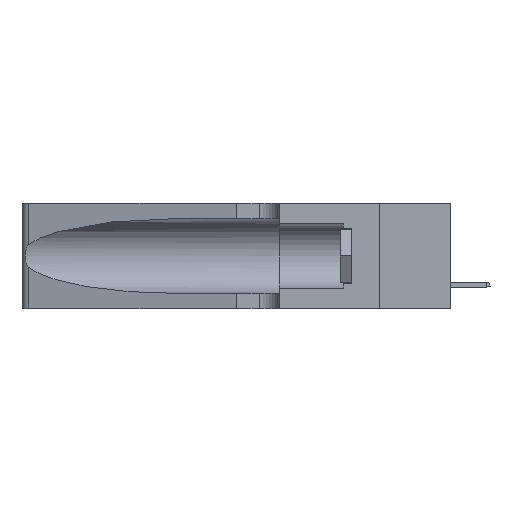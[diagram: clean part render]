
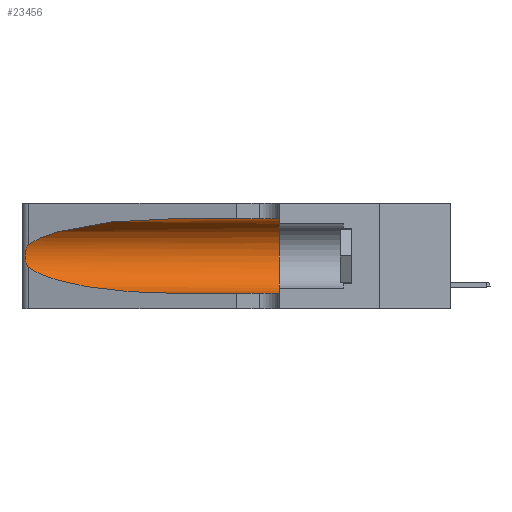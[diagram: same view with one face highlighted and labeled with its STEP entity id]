
A CAD part, left-side view. The second image highlights one B-rep face of the part: STEP entity #23456.
In plain terms, the highlighted cylindrical face has radius 3.308 mm (diameter 6.617 mm), a partial arc.
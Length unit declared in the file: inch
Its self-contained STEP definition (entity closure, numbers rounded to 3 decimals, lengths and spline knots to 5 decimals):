
#141 = CARTESIAN_POINT ( 'NONE',  ( 0.25555, 1.22994, 0.2215 ) ) ;
#647 = CARTESIAN_POINT ( 'NONE',  ( 0.18966, 0.96281, 0.31525 ) ) ;
#2506 = DIRECTION ( 'NONE',  ( 0., -1., 0. ) ) ;
#3282 = AXIS2_PLACEMENT_3D ( 'NONE', #23317, #33966, #10774 ) ;
#3407 = CARTESIAN_POINT ( 'NONE',  ( 0.1305, 1.61858, 0.31525 ) ) ;
#4563 = CARTESIAN_POINT ( 'NONE',  ( 0.1305, 0.72297, 0.31525 ) ) ;
#7041 = CARTESIAN_POINT ( 'NONE',  ( 0.25555, 1.22993, 0.14849 ) ) ;
#7470 = DIRECTION ( 'NONE',  ( 0., 1., 0. ) ) ;
#8236 =( BOUNDED_CURVE ( )  B_SPLINE_CURVE ( 3, ( #4563, #647, #25328, #32719 ),
 .UNSPECIFIED., .F., .T. ) 
 B_SPLINE_CURVE_WITH_KNOTS ( ( 4, 4 ),
 ( 1.5708, 2.84003 ),
 .UNSPECIFIED. ) 
 CURVE ( )  GEOMETRIC_REPRESENTATION_ITEM ( )  RATIONAL_B_SPLINE_CURVE ( ( 1., 0.87, 0.87, 1. ) ) 
 REPRESENTATION_ITEM ( '' )  );
#8951 = ORIENTED_EDGE ( 'NONE', *, *, #14576, .T. ) ;
#10418 = CARTESIAN_POINT ( 'NONE',  ( 0.1305, 1.61858, 0.05475 ) ) ;
#10507 = CARTESIAN_POINT ( 'NONE',  ( 0.25789, 1.23486, 0.15765 ) ) ;
#10774 = DIRECTION ( 'NONE',  ( 0., 0., -1. ) ) ;
#11769 = CARTESIAN_POINT ( 'NONE',  ( 0.1305, 0.35, 0.31525 ) ) ;
#13857 = CARTESIAN_POINT ( 'NONE',  ( 0.25487, 1.22718, 0.14631 ) ) ;
#13956 = CARTESIAN_POINT ( 'NONE',  ( 0.25856, 1.23593, 0.16098 ) ) ;
#14417 = AXIS2_PLACEMENT_3D ( 'NONE', #35677, #7470, #35895 ) ;
#14576 = EDGE_CURVE ( 'NONE', #36772, #32046, #20789, .T. ) ;
#14887 = CARTESIAN_POINT ( 'NONE',  ( 0.25487, 1.22718, 0.22369 ) ) ;
#15373 = CARTESIAN_POINT ( 'NONE',  ( 0.1305, 0.72297, 0.05475 ) ) ;
#15711 = CARTESIAN_POINT ( 'NONE',  ( 0.25487, 1.22718, 0.14631 ) ) ;
#16913 = CARTESIAN_POINT ( 'NONE',  ( 0.1305, 0.72297, 0.31525 ) ) ;
#17867 = VECTOR ( 'NONE', #2506, 39.37008 ) ;
#18005 = ORIENTED_EDGE ( 'NONE', *, *, #28776, .T. ) ;
#18934 = VECTOR ( 'NONE', #21506, 39.37008 ) ;
#19103 = EDGE_CURVE ( 'NONE', #30252, #42245, #34595, .T. ) ;
#19390 = CARTESIAN_POINT ( 'NONE',  ( 0.1305, 0.72297, 0.05475 ) ) ;
#19509 = EDGE_LOOP ( 'NONE', ( #20679, #8951, #19582, #18005, #43966, #21926 ) ) ;
#19582 = ORIENTED_EDGE ( 'NONE', *, *, #23451, .T. ) ;
#20611 = EDGE_CURVE ( 'NONE', #30252, #36772, #8236, .T. ) ;
#20679 = ORIENTED_EDGE ( 'NONE', *, *, #20611, .T. ) ;
#20789 = B_SPLINE_CURVE_WITH_KNOTS ( 'NONE', 3,
 ( #14887, #141, #21116, #28063, #43056, #42387, #21339, #22646, #42831, #13956, #10507, #24604, #7041, #35237 ),
 .UNSPECIFIED., .F., .F.,
 ( 4, 2, 2, 2, 2, 2, 4 ),
 ( 0., 0.00027, 0.00053, 0.00107, 0.0016, 0.00187, 0.00214 ),
 .UNSPECIFIED. ) ;
#21116 = CARTESIAN_POINT ( 'NONE',  ( 0.25639, 1.23184, 0.21858 ) ) ;
#21339 = CARTESIAN_POINT ( 'NONE',  ( 0.26075, 1.23896, 0.19203 ) ) ;
#21506 = DIRECTION ( 'NONE',  ( 0., -1., 0. ) ) ;
#21926 = ORIENTED_EDGE ( 'NONE', *, *, #19103, .F. ) ;
#22646 = CARTESIAN_POINT ( 'NONE',  ( 0.26075, 1.23896, 0.178 ) ) ;
#23317 = CARTESIAN_POINT ( 'NONE',  ( 0.1305, 1.61858, 0.185 ) ) ;
#23451 = EDGE_CURVE ( 'NONE', #32046, #23654, #28899, .T. ) ;
#23456 = ADVANCED_FACE ( 'NONE', ( #26337 ), #27015, .F. ) ;
#23654 = VERTEX_POINT ( 'NONE', #15373 ) ;
#24604 = CARTESIAN_POINT ( 'NONE',  ( 0.25639, 1.23186, 0.15144 ) ) ;
#25328 = CARTESIAN_POINT ( 'NONE',  ( 0.2373, 1.15595, 0.28018 ) ) ;
#26337 = FACE_OUTER_BOUND ( 'NONE', #19509, .T. ) ;
#27015 = CYLINDRICAL_SURFACE ( 'NONE', #3282, 0.13025 ) ;
#28063 = CARTESIAN_POINT ( 'NONE',  ( 0.25787, 1.23484, 0.2124 ) ) ;
#28776 = EDGE_CURVE ( 'NONE', #23654, #35247, #42076, .T. ) ;
#28899 =( BOUNDED_CURVE ( )  B_SPLINE_CURVE ( 3, ( #15711, #29810, #43862, #19390 ),
 .UNSPECIFIED., .F., .T. ) 
 B_SPLINE_CURVE_WITH_KNOTS ( ( 4, 4 ),
 ( 3.44316, 4.71239 ),
 .UNSPECIFIED. ) 
 CURVE ( )  GEOMETRIC_REPRESENTATION_ITEM ( )  RATIONAL_B_SPLINE_CURVE ( ( 1., 0.87, 0.87, 1. ) ) 
 REPRESENTATION_ITEM ( '' )  );
#29810 = CARTESIAN_POINT ( 'NONE',  ( 0.2373, 1.15595, 0.08982 ) ) ;
#30252 = VERTEX_POINT ( 'NONE', #16913 ) ;
#31770 = CARTESIAN_POINT ( 'NONE',  ( 0.25487, 1.22718, 0.22369 ) ) ;
#32046 = VERTEX_POINT ( 'NONE', #13857 ) ;
#32719 = CARTESIAN_POINT ( 'NONE',  ( 0.25487, 1.22718, 0.22369 ) ) ;
#33966 = DIRECTION ( 'NONE',  ( 0., -1., 0. ) ) ;
#34595 = LINE ( 'NONE', #3407, #17867 ) ;
#35237 = CARTESIAN_POINT ( 'NONE',  ( 0.25487, 1.22718, 0.14631 ) ) ;
#35247 = VERTEX_POINT ( 'NONE', #43340 ) ;
#35677 = CARTESIAN_POINT ( 'NONE',  ( 0.1305, 0.35, 0.185 ) ) ;
#35895 = DIRECTION ( 'NONE',  ( 0., 0., 1. ) ) ;
#36772 = VERTEX_POINT ( 'NONE', #31770 ) ;
#38761 = CIRCLE ( 'NONE', #14417, 0.13025 ) ;
#39361 = EDGE_CURVE ( 'NONE', #42245, #35247, #38761, .T. ) ;
#42076 = LINE ( 'NONE', #10418, #18934 ) ;
#42245 = VERTEX_POINT ( 'NONE', #11769 ) ;
#42387 = CARTESIAN_POINT ( 'NONE',  ( 0.26018, 1.23835, 0.19895 ) ) ;
#42831 = CARTESIAN_POINT ( 'NONE',  ( 0.26017, 1.23833, 0.17102 ) ) ;
#43056 = CARTESIAN_POINT ( 'NONE',  ( 0.25854, 1.2359, 0.20912 ) ) ;
#43340 = CARTESIAN_POINT ( 'NONE',  ( 0.1305, 0.35, 0.05475 ) ) ;
#43862 = CARTESIAN_POINT ( 'NONE',  ( 0.18966, 0.96281, 0.05475 ) ) ;
#43966 = ORIENTED_EDGE ( 'NONE', *, *, #39361, .F. ) ;
